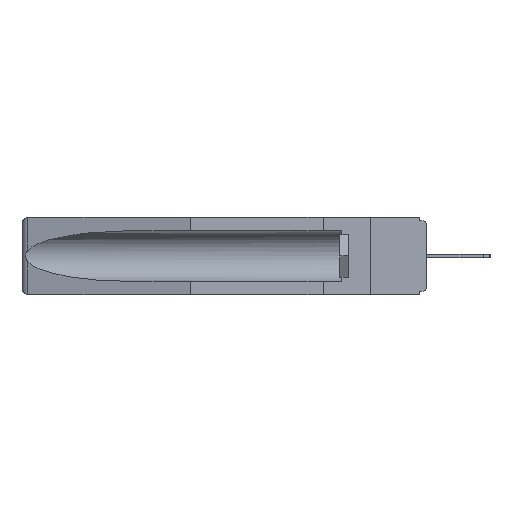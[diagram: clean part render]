
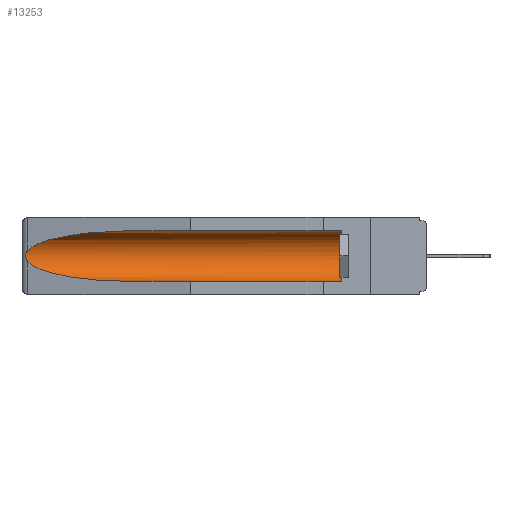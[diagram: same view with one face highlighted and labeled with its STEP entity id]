
A CAD part, left-side view. The second image highlights one B-rep face of the part: STEP entity #13253.
In plain terms, the highlighted cylindrical face has radius 2.857 mm (diameter 5.715 mm), a partial arc.
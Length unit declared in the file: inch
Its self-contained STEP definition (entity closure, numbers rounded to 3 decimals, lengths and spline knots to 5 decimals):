
#330 =( BOUNDED_CURVE ( )  B_SPLINE_CURVE ( 3, ( #6246, #6306, #17665, #6572 ),
 .UNSPECIFIED., .F., .F. ) 
 B_SPLINE_CURVE_WITH_KNOTS ( ( 4, 4 ),
 ( 0.1948, 1.5708 ),
 .UNSPECIFIED. ) 
 CURVE ( )  GEOMETRIC_REPRESENTATION_ITEM ( )  RATIONAL_B_SPLINE_CURVE ( ( 1., 0.848, 0.848, 1. ) ) 
 REPRESENTATION_ITEM ( '' )  );
#768 = EDGE_CURVE ( 'NONE', #8691, #21633, #3181, .T. ) ;
#1176 = CARTESIAN_POINT ( 'NONE',  ( 0.26597, 1.52961, -0.15275 ) ) ;
#1225 = CARTESIAN_POINT ( 'NONE',  ( 0.26537, 1.52718, -0.19328 ) ) ;
#1320 = ORIENTED_EDGE ( 'NONE', *, *, #3695, .T. ) ;
#1564 = CARTESIAN_POINT ( 'NONE',  ( 0.155, -0.30754, -0.059 ) ) ;
#2907 = CARTESIAN_POINT ( 'NONE',  ( 0.155, 0.126, -0.1715 ) ) ;
#3181 = LINE ( 'NONE', #1564, #19331 ) ;
#3189 = CARTESIAN_POINT ( 'NONE',  ( 0.26537, 1.52718, -0.14972 ) ) ;
#3377 = CARTESIAN_POINT ( 'NONE',  ( 0.26654, 1.53092, -0.15636 ) ) ;
#3695 = EDGE_CURVE ( 'NONE', #7953, #19400, #330, .T. ) ;
#5077 = DIRECTION ( 'NONE',  ( 0., 0., 1. ) ) ;
#5540 = CARTESIAN_POINT ( 'NONE',  ( 0.2675, 1.53308, -0.16763 ) ) ;
#6157 = CARTESIAN_POINT ( 'NONE',  ( 0.155, 1.07973, -0.284 ) ) ;
#6246 = CARTESIAN_POINT ( 'NONE',  ( 0.26537, 1.52718, -0.19328 ) ) ;
#6306 = CARTESIAN_POINT ( 'NONE',  ( 0.25451, 1.48313, -0.24835 ) ) ;
#6572 = CARTESIAN_POINT ( 'NONE',  ( 0.155, 1.07973, -0.284 ) ) ;
#6777 = CARTESIAN_POINT ( 'NONE',  ( 0.26537, 1.52718, -0.14972 ) ) ;
#7492 = CARTESIAN_POINT ( 'NONE',  ( 0.155, -0.30754, -0.284 ) ) ;
#7730 = CARTESIAN_POINT ( 'NONE',  ( 0.2673, 1.53269, -0.17917 ) ) ;
#7939 = CARTESIAN_POINT ( 'NONE',  ( 0.155, 1.07973, -0.059 ) ) ;
#7953 = VERTEX_POINT ( 'NONE', #1225 ) ;
#8069 = ORIENTED_EDGE ( 'NONE', *, *, #9798, .T. ) ;
#8316 = CARTESIAN_POINT ( 'NONE',  ( 0.155, -0.30754, -0.1715 ) ) ;
#8691 = VERTEX_POINT ( 'NONE', #12339 ) ;
#9669 = CARTESIAN_POINT ( 'NONE',  ( 0.25451, 1.48313, -0.09465 ) ) ;
#9798 = EDGE_CURVE ( 'NONE', #21633, #20716, #24283, .T. ) ;
#9896 = CARTESIAN_POINT ( 'NONE',  ( 0.26597, 1.5296, -0.19026 ) ) ;
#11303 = CYLINDRICAL_SURFACE ( 'NONE', #15486, 0.1125 ) ;
#11749 = CARTESIAN_POINT ( 'NONE',  ( 0.155, 1.07973, -0.059 ) ) ;
#12000 = B_SPLINE_CURVE_WITH_KNOTS ( 'NONE', 3,
 ( #3189, #1176, #3377, #18120, #5540, #20222, #7730, #22310, #9896, #24389 ),
 .UNSPECIFIED., .F., .F.,
 ( 4, 2, 2, 2, 4 ),
 ( 0., 0.00029, 0.00058, 0.00087, 0.00117 ),
 .UNSPECIFIED. ) ;
#12339 = CARTESIAN_POINT ( 'NONE',  ( 0.155, 0.126, -0.059 ) ) ;
#12683 = CIRCLE ( 'NONE', #18817, 0.1125 ) ;
#13253 = ADVANCED_FACE ( 'NONE', ( #18091 ), #11303, .F. ) ;
#14626 = DIRECTION ( 'NONE',  ( 0., 0., 1. ) ) ;
#14846 = CARTESIAN_POINT ( 'NONE',  ( 0.155, 0.126, -0.284 ) ) ;
#15486 = AXIS2_PLACEMENT_3D ( 'NONE', #8316, #22898, #14626 ) ;
#15811 = CARTESIAN_POINT ( 'NONE',  ( 0.21114, 1.30732, -0.059 ) ) ;
#16969 = VERTEX_POINT ( 'NONE', #14846 ) ;
#17665 = CARTESIAN_POINT ( 'NONE',  ( 0.21114, 1.30732, -0.284 ) ) ;
#17675 = DIRECTION ( 'NONE',  ( 0., -1., 0. ) ) ;
#18091 = FACE_OUTER_BOUND ( 'NONE', #19899, .T. ) ;
#18120 = CARTESIAN_POINT ( 'NONE',  ( 0.2673, 1.5327, -0.16383 ) ) ;
#18817 = AXIS2_PLACEMENT_3D ( 'NONE', #2907, #17675, #5077 ) ;
#19331 = VECTOR ( 'NONE', #26781, 39.37008 ) ;
#19400 = VERTEX_POINT ( 'NONE', #6157 ) ;
#19899 = EDGE_LOOP ( 'NONE', ( #8069, #22074, #1320, #20580, #19900, #22651 ) ) ;
#19900 = ORIENTED_EDGE ( 'NONE', *, *, #25004, .T. ) ;
#19987 = DIRECTION ( 'NONE',  ( 0., 1., 0. ) ) ;
#20222 = CARTESIAN_POINT ( 'NONE',  ( 0.2675, 1.53308, -0.17534 ) ) ;
#20580 = ORIENTED_EDGE ( 'NONE', *, *, #21494, .F. ) ;
#20716 = VERTEX_POINT ( 'NONE', #6777 ) ;
#21494 = EDGE_CURVE ( 'NONE', #16969, #19400, #27188, .T. ) ;
#21633 = VERTEX_POINT ( 'NONE', #7939 ) ;
#21688 = VECTOR ( 'NONE', #19987, 39.37008 ) ;
#22074 = ORIENTED_EDGE ( 'NONE', *, *, #22556, .T. ) ;
#22310 = CARTESIAN_POINT ( 'NONE',  ( 0.26655, 1.53094, -0.18657 ) ) ;
#22556 = EDGE_CURVE ( 'NONE', #20716, #7953, #12000, .T. ) ;
#22651 = ORIENTED_EDGE ( 'NONE', *, *, #768, .T. ) ;
#22898 = DIRECTION ( 'NONE',  ( 0., 1., 0. ) ) ;
#24283 =( BOUNDED_CURVE ( )  B_SPLINE_CURVE ( 3, ( #11749, #15811, #9669, #26245 ),
 .UNSPECIFIED., .F., .F. ) 
 B_SPLINE_CURVE_WITH_KNOTS ( ( 4, 4 ),
 ( 4.71239, 6.08839 ),
 .UNSPECIFIED. ) 
 CURVE ( )  GEOMETRIC_REPRESENTATION_ITEM ( )  RATIONAL_B_SPLINE_CURVE ( ( 1., 0.848, 0.848, 1. ) ) 
 REPRESENTATION_ITEM ( '' )  );
#24389 = CARTESIAN_POINT ( 'NONE',  ( 0.26537, 1.52718, -0.19328 ) ) ;
#25004 = EDGE_CURVE ( 'NONE', #16969, #8691, #12683, .T. ) ;
#26245 = CARTESIAN_POINT ( 'NONE',  ( 0.26537, 1.52718, -0.14972 ) ) ;
#26781 = DIRECTION ( 'NONE',  ( 0., 1., 0. ) ) ;
#27188 = LINE ( 'NONE', #7492, #21688 ) ;
